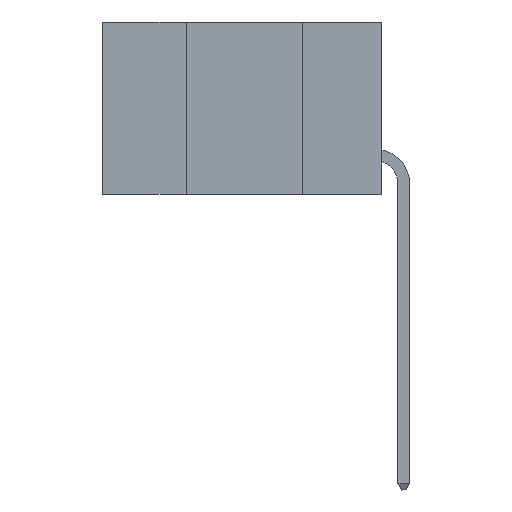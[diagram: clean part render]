
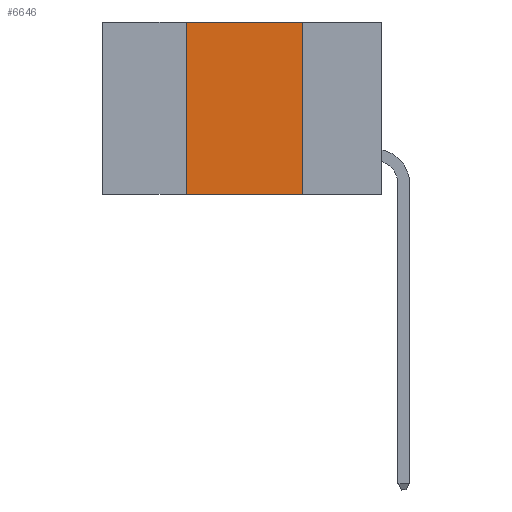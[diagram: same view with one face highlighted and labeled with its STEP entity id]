
A CAD part, left-side view. The second image highlights one B-rep face of the part: STEP entity #6646.
In plain terms, the highlighted planar face has unit normal (-1, 0, 0).
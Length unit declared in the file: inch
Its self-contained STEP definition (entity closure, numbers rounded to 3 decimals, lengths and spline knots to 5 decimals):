
#330 = ORIENTED_EDGE ( 'NONE', *, *, #12358, .F. ) ;
#1039 = VERTEX_POINT ( 'NONE', #16310 ) ;
#1106 = CARTESIAN_POINT ( 'NONE',  ( 0., 0.6, 0. ) ) ;
#1818 = LINE ( 'NONE', #10451, #14540 ) ;
#2647 = ORIENTED_EDGE ( 'NONE', *, *, #7331, .F. ) ;
#3042 = CARTESIAN_POINT ( 'NONE',  ( 0., 0.6, -0.37 ) ) ;
#3231 = CARTESIAN_POINT ( 'NONE',  ( 0., 0.42, 0. ) ) ;
#3423 = ORIENTED_EDGE ( 'NONE', *, *, #10532, .T. ) ;
#3443 = DIRECTION ( 'NONE',  ( 0., -1., 0. ) ) ;
#3710 = VECTOR ( 'NONE', #7933, 39.37008 ) ;
#4865 = EDGE_CURVE ( 'NONE', #8603, #1039, #10750, .T. ) ;
#5489 = AXIS2_PLACEMENT_3D ( 'NONE', #5549, #5841, #5665 ) ;
#5549 = CARTESIAN_POINT ( 'NONE',  ( 0., 0.6, 0. ) ) ;
#5665 = DIRECTION ( 'NONE',  ( 0., 0., -1. ) ) ;
#5819 = VECTOR ( 'NONE', #3443, 39.37008 ) ;
#5841 = DIRECTION ( 'NONE',  ( 1., 0., 0. ) ) ;
#6646 = ADVANCED_FACE ( 'NONE', ( #16250 ), #9563, .F. ) ;
#7290 = VECTOR ( 'NONE', #9048, 39.37008 ) ;
#7331 = EDGE_CURVE ( 'NONE', #1039, #12040, #9070, .T. ) ;
#7575 = CARTESIAN_POINT ( 'NONE',  ( 0., 0.42, -0.37 ) ) ;
#7933 = DIRECTION ( 'NONE',  ( 0., 0., -1. ) ) ;
#8073 = LINE ( 'NONE', #3042, #5819 ) ;
#8603 = VERTEX_POINT ( 'NONE', #3231 ) ;
#9048 = DIRECTION ( 'NONE',  ( 0., -1., 0. ) ) ;
#9070 = LINE ( 'NONE', #14351, #3710 ) ;
#9563 = PLANE ( 'NONE',  #5489 ) ;
#10426 = VERTEX_POINT ( 'NONE', #7575 ) ;
#10451 = CARTESIAN_POINT ( 'NONE',  ( 0., 0.42, 0. ) ) ;
#10532 = EDGE_CURVE ( 'NONE', #10426, #12040, #8073, .T. ) ;
#10750 = LINE ( 'NONE', #1106, #7290 ) ;
#12040 = VERTEX_POINT ( 'NONE', #13447 ) ;
#12358 = EDGE_CURVE ( 'NONE', #10426, #8603, #1818, .T. ) ;
#13447 = CARTESIAN_POINT ( 'NONE',  ( 0., 0.17, -0.37 ) ) ;
#14351 = CARTESIAN_POINT ( 'NONE',  ( 0., 0.17, 0. ) ) ;
#14431 = EDGE_LOOP ( 'NONE', ( #2647, #14547, #330, #3423 ) ) ;
#14481 = DIRECTION ( 'NONE',  ( 0., 0., 1. ) ) ;
#14540 = VECTOR ( 'NONE', #14481, 39.37008 ) ;
#14547 = ORIENTED_EDGE ( 'NONE', *, *, #4865, .F. ) ;
#16250 = FACE_OUTER_BOUND ( 'NONE', #14431, .T. ) ;
#16310 = CARTESIAN_POINT ( 'NONE',  ( 0., 0.17, 0. ) ) ;
